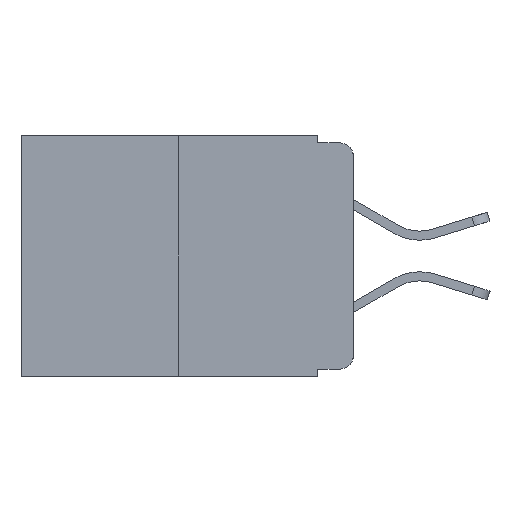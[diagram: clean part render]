
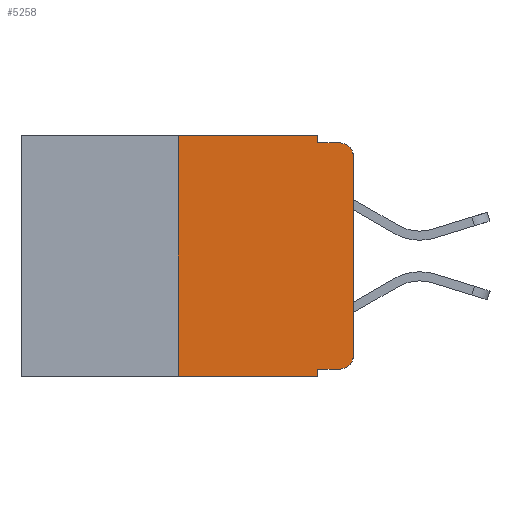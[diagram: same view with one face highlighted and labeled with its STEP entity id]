
A CAD part, left-side view. The second image highlights one B-rep face of the part: STEP entity #5258.
In plain terms, the highlighted planar face has unit normal (-1, 0, 0).
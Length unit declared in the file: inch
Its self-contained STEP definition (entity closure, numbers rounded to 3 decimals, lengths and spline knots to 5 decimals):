
#108 = CARTESIAN_POINT ( 'NONE',  ( 0., 0.051, -0.333 ) ) ;
#354 = PLANE ( 'NONE',  #11449 ) ;
#484 = VECTOR ( 'NONE', #3714, 39.37008 ) ;
#828 = VERTEX_POINT ( 'NONE', #5916 ) ;
#848 = CARTESIAN_POINT ( 'NONE',  ( 0., 0.473, 0. ) ) ;
#1106 = AXIS2_PLACEMENT_3D ( 'NONE', #7174, #14477, #12000 ) ;
#1283 = LINE ( 'NONE', #7388, #2341 ) ;
#1431 = VERTEX_POINT ( 'NONE', #15215 ) ;
#1655 = EDGE_LOOP ( 'NONE', ( #10885, #14539, #9007, #6291, #4896, #5402, #6725, #5687, #12048, #7116 ) ) ;
#2047 = VERTEX_POINT ( 'NONE', #11928 ) ;
#2143 = DIRECTION ( 'NONE',  ( 0., 0., 1. ) ) ;
#2341 = VECTOR ( 'NONE', #12054, 39.37008 ) ;
#2431 = VECTOR ( 'NONE', #12649, 39.37008 ) ;
#3174 = LINE ( 'NONE', #13888, #4870 ) ;
#3353 = AXIS2_PLACEMENT_3D ( 'NONE', #12949, #9004, #12860 ) ;
#3439 = VERTEX_POINT ( 'NONE', #12327 ) ;
#3477 = CARTESIAN_POINT ( 'NONE',  ( 0., 0., 0. ) ) ;
#3714 = DIRECTION ( 'NONE',  ( 0., 0., 1. ) ) ;
#3750 = FACE_OUTER_BOUND ( 'NONE', #1655, .T. ) ;
#3810 = LINE ( 'NONE', #108, #8925 ) ;
#4125 = LINE ( 'NONE', #8969, #7935 ) ;
#4584 = VERTEX_POINT ( 'NONE', #6810 ) ;
#4672 = CARTESIAN_POINT ( 'NONE',  ( 0., 0.25, 0. ) ) ;
#4870 = VECTOR ( 'NONE', #10088, 39.37008 ) ;
#4896 = ORIENTED_EDGE ( 'NONE', *, *, #15153, .F. ) ;
#5024 = CARTESIAN_POINT ( 'NONE',  ( 0., 0., -0.03 ) ) ;
#5087 = DIRECTION ( 'NONE',  ( 0., -1., 0. ) ) ;
#5210 = DIRECTION ( 'NONE',  ( 0., 0., -1. ) ) ;
#5255 = VERTEX_POINT ( 'NONE', #5024 ) ;
#5258 = ADVANCED_FACE ( 'NONE', ( #3750 ), #354, .F. ) ;
#5337 = EDGE_CURVE ( 'NONE', #13513, #3439, #3174, .T. ) ;
#5402 = ORIENTED_EDGE ( 'NONE', *, *, #13520, .F. ) ;
#5650 = CIRCLE ( 'NONE', #1106, 0.02 ) ;
#5687 = ORIENTED_EDGE ( 'NONE', *, *, #15421, .F. ) ;
#5705 = EDGE_CURVE ( 'NONE', #12262, #15042, #1283, .T. ) ;
#5731 = EDGE_CURVE ( 'NONE', #2047, #14866, #3810, .T. ) ;
#5893 = EDGE_CURVE ( 'NONE', #1431, #12262, #4125, .T. ) ;
#5916 = CARTESIAN_POINT ( 'NONE',  ( 0., 0., -0.313 ) ) ;
#6214 = EDGE_CURVE ( 'NONE', #14866, #828, #13745, .T. ) ;
#6291 = ORIENTED_EDGE ( 'NONE', *, *, #5893, .F. ) ;
#6388 = CARTESIAN_POINT ( 'NONE',  ( 0., 0.051, -0.01 ) ) ;
#6426 = EDGE_CURVE ( 'NONE', #5255, #15042, #5650, .T. ) ;
#6471 = LINE ( 'NONE', #14654, #10778 ) ;
#6725 = ORIENTED_EDGE ( 'NONE', *, *, #5337, .T. ) ;
#6810 = CARTESIAN_POINT ( 'NONE',  ( 0., 0.25, 0. ) ) ;
#7116 = ORIENTED_EDGE ( 'NONE', *, *, #6214, .T. ) ;
#7174 = CARTESIAN_POINT ( 'NONE',  ( 0., 0.02, -0.03 ) ) ;
#7388 = CARTESIAN_POINT ( 'NONE',  ( 0., 0.051, -0.01 ) ) ;
#7935 = VECTOR ( 'NONE', #13799, 39.37008 ) ;
#8321 = LINE ( 'NONE', #4672, #484 ) ;
#8523 = CARTESIAN_POINT ( 'NONE',  ( 0., 0.473, 0. ) ) ;
#8540 = EDGE_CURVE ( 'NONE', #828, #5255, #12043, .T. ) ;
#8824 = DIRECTION ( 'NONE',  ( 1., 0., 0. ) ) ;
#8925 = VECTOR ( 'NONE', #5087, 39.37008 ) ;
#8969 = CARTESIAN_POINT ( 'NONE',  ( 0., 0.051, 0. ) ) ;
#9004 = DIRECTION ( 'NONE',  ( -1., 0., 0. ) ) ;
#9007 = ORIENTED_EDGE ( 'NONE', *, *, #5705, .F. ) ;
#9752 = CARTESIAN_POINT ( 'NONE',  ( 0., 0.25, -0.343 ) ) ;
#10088 = DIRECTION ( 'NONE',  ( 0., -1., 0. ) ) ;
#10445 = LINE ( 'NONE', #848, #2431 ) ;
#10778 = VECTOR ( 'NONE', #5210, 39.37008 ) ;
#10885 = ORIENTED_EDGE ( 'NONE', *, *, #8540, .T. ) ;
#11213 = DIRECTION ( 'NONE',  ( 0., 0., -1. ) ) ;
#11449 = AXIS2_PLACEMENT_3D ( 'NONE', #8523, #8824, #11213 ) ;
#11928 = CARTESIAN_POINT ( 'NONE',  ( 0., 0.051, -0.333 ) ) ;
#12000 = DIRECTION ( 'NONE',  ( 0., 0., -1. ) ) ;
#12043 = LINE ( 'NONE', #3477, #15184 ) ;
#12048 = ORIENTED_EDGE ( 'NONE', *, *, #5731, .T. ) ;
#12054 = DIRECTION ( 'NONE',  ( 0., -1., 0. ) ) ;
#12262 = VERTEX_POINT ( 'NONE', #6388 ) ;
#12327 = CARTESIAN_POINT ( 'NONE',  ( 0., 0.051, -0.343 ) ) ;
#12503 = CARTESIAN_POINT ( 'NONE',  ( 0., 0.02, -0.01 ) ) ;
#12649 = DIRECTION ( 'NONE',  ( 0., -1., 0. ) ) ;
#12860 = DIRECTION ( 'NONE',  ( 0., 0., -1. ) ) ;
#12949 = CARTESIAN_POINT ( 'NONE',  ( 0., 0.02, -0.313 ) ) ;
#13064 = CARTESIAN_POINT ( 'NONE',  ( 0., 0.02, -0.333 ) ) ;
#13513 = VERTEX_POINT ( 'NONE', #9752 ) ;
#13520 = EDGE_CURVE ( 'NONE', #13513, #4584, #8321, .T. ) ;
#13745 = CIRCLE ( 'NONE', #3353, 0.02 ) ;
#13799 = DIRECTION ( 'NONE',  ( 0., 0., -1. ) ) ;
#13888 = CARTESIAN_POINT ( 'NONE',  ( 0., 0.473, -0.343 ) ) ;
#14477 = DIRECTION ( 'NONE',  ( -1., 0., 0. ) ) ;
#14539 = ORIENTED_EDGE ( 'NONE', *, *, #6426, .T. ) ;
#14654 = CARTESIAN_POINT ( 'NONE',  ( 0., 0.051, 0. ) ) ;
#14866 = VERTEX_POINT ( 'NONE', #13064 ) ;
#15042 = VERTEX_POINT ( 'NONE', #12503 ) ;
#15153 = EDGE_CURVE ( 'NONE', #4584, #1431, #10445, .T. ) ;
#15184 = VECTOR ( 'NONE', #2143, 39.37008 ) ;
#15215 = CARTESIAN_POINT ( 'NONE',  ( 0., 0.051, 0. ) ) ;
#15421 = EDGE_CURVE ( 'NONE', #2047, #3439, #6471, .T. ) ;
